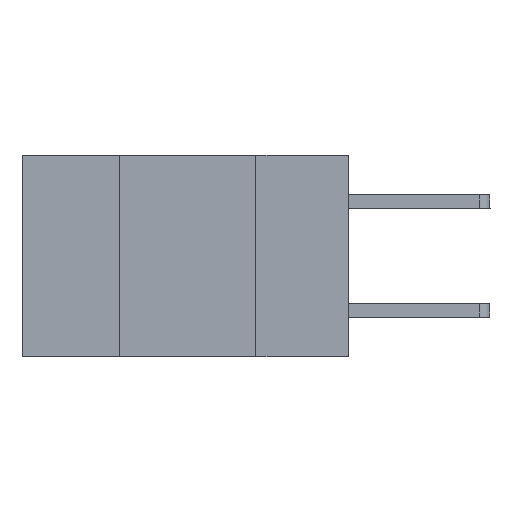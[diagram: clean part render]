
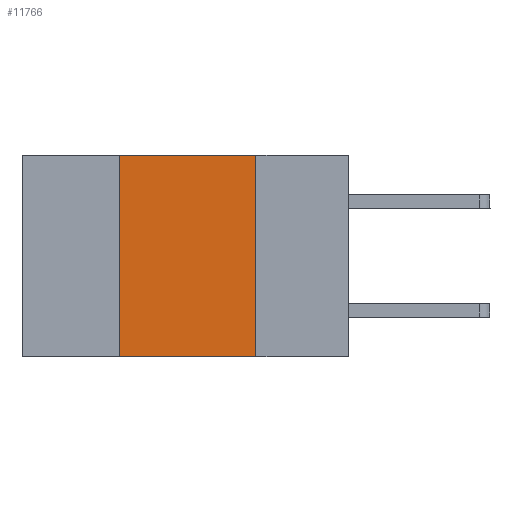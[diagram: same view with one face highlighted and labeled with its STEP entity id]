
A CAD part, left-side view. The second image highlights one B-rep face of the part: STEP entity #11766.
In plain terms, the highlighted planar face has unit normal (-1, 0, 0).
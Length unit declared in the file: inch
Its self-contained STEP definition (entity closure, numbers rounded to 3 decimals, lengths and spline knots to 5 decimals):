
#500 = VECTOR ( 'NONE', #5238, 39.37008 ) ;
#675 = CARTESIAN_POINT ( 'NONE',  ( 0., 0.17, 0. ) ) ;
#1027 = DIRECTION ( 'NONE',  ( 1., 0., 0. ) ) ;
#1212 = CARTESIAN_POINT ( 'NONE',  ( 0., 0.6, 0. ) ) ;
#1324 = EDGE_CURVE ( 'NONE', #3021, #9691, #11358, .T. ) ;
#1824 = CARTESIAN_POINT ( 'NONE',  ( 0., 0.6, 0. ) ) ;
#2113 = LINE ( 'NONE', #1212, #6367 ) ;
#2404 = ORIENTED_EDGE ( 'NONE', *, *, #2826, .F. ) ;
#2534 = CARTESIAN_POINT ( 'NONE',  ( 0., 0.42, -0.37 ) ) ;
#2673 = CARTESIAN_POINT ( 'NONE',  ( 0., 0.42, 0. ) ) ;
#2826 = EDGE_CURVE ( 'NONE', #9056, #9691, #8789, .T. ) ;
#3021 = VERTEX_POINT ( 'NONE', #2534 ) ;
#4002 = VECTOR ( 'NONE', #8871, 39.37008 ) ;
#4468 = EDGE_CURVE ( 'NONE', #5520, #9056, #2113, .T. ) ;
#4817 = CARTESIAN_POINT ( 'NONE',  ( 0., 0.6, -0.37 ) ) ;
#4861 = DIRECTION ( 'NONE',  ( 0., -1., 0. ) ) ;
#5077 = CARTESIAN_POINT ( 'NONE',  ( 0., 0.17, 0. ) ) ;
#5238 = DIRECTION ( 'NONE',  ( 0., 0., -1. ) ) ;
#5403 = DIRECTION ( 'NONE',  ( 0., 0., -1. ) ) ;
#5520 = VERTEX_POINT ( 'NONE', #6091 ) ;
#5556 = ORIENTED_EDGE ( 'NONE', *, *, #1324, .T. ) ;
#5581 = ORIENTED_EDGE ( 'NONE', *, *, #5590, .F. ) ;
#5590 = EDGE_CURVE ( 'NONE', #3021, #5520, #9064, .T. ) ;
#6091 = CARTESIAN_POINT ( 'NONE',  ( 0., 0.42, 0. ) ) ;
#6367 = VECTOR ( 'NONE', #4861, 39.37008 ) ;
#7864 = EDGE_LOOP ( 'NONE', ( #2404, #9014, #5581, #5556 ) ) ;
#8095 = VECTOR ( 'NONE', #8497, 39.37008 ) ;
#8497 = DIRECTION ( 'NONE',  ( 0., -1., 0. ) ) ;
#8789 = LINE ( 'NONE', #675, #500 ) ;
#8871 = DIRECTION ( 'NONE',  ( 0., 0., 1. ) ) ;
#9014 = ORIENTED_EDGE ( 'NONE', *, *, #4468, .F. ) ;
#9056 = VERTEX_POINT ( 'NONE', #5077 ) ;
#9064 = LINE ( 'NONE', #2673, #4002 ) ;
#9272 = PLANE ( 'NONE',  #10988 ) ;
#9691 = VERTEX_POINT ( 'NONE', #11857 ) ;
#10988 = AXIS2_PLACEMENT_3D ( 'NONE', #1824, #1027, #5403 ) ;
#11168 = FACE_OUTER_BOUND ( 'NONE', #7864, .T. ) ;
#11358 = LINE ( 'NONE', #4817, #8095 ) ;
#11766 = ADVANCED_FACE ( 'NONE', ( #11168 ), #9272, .F. ) ;
#11857 = CARTESIAN_POINT ( 'NONE',  ( 0., 0.17, -0.37 ) ) ;
